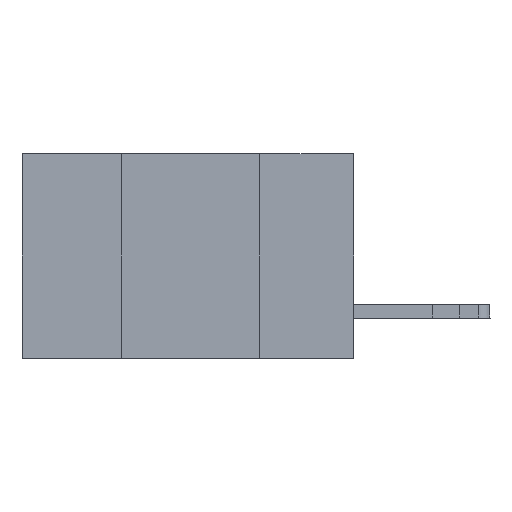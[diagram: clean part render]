
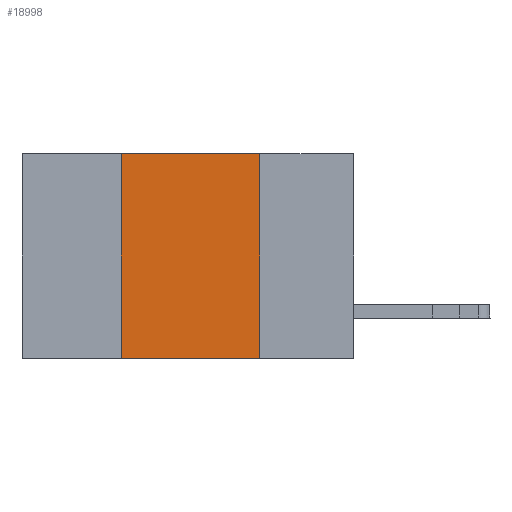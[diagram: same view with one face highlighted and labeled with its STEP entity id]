
A CAD part, left-side view. The second image highlights one B-rep face of the part: STEP entity #18998.
In plain terms, the highlighted planar face has unit normal (-1, 0, 0).
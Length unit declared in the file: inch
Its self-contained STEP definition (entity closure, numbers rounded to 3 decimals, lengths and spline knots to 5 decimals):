
#473 = LINE ( 'NONE', #11415, #4688 ) ;
#1109 = EDGE_CURVE ( 'NONE', #12487, #18572, #7419, .T. ) ;
#1153 = VERTEX_POINT ( 'NONE', #19826 ) ;
#2046 = ORIENTED_EDGE ( 'NONE', *, *, #14550, .T. ) ;
#2418 = CARTESIAN_POINT ( 'NONE',  ( 0., 0.6, -0.37 ) ) ;
#3760 = EDGE_LOOP ( 'NONE', ( #18674, #7766, #18654, #2046 ) ) ;
#4688 = VECTOR ( 'NONE', #9713, 39.37008 ) ;
#5817 = CARTESIAN_POINT ( 'NONE',  ( 0., 0.6, 0. ) ) ;
#6160 = CARTESIAN_POINT ( 'NONE',  ( 0., 0.17, 0. ) ) ;
#6747 = CARTESIAN_POINT ( 'NONE',  ( 0., 0.42, 0. ) ) ;
#7419 = LINE ( 'NONE', #18653, #14099 ) ;
#7720 = FACE_OUTER_BOUND ( 'NONE', #3760, .T. ) ;
#7766 = ORIENTED_EDGE ( 'NONE', *, *, #1109, .F. ) ;
#9285 = DIRECTION ( 'NONE',  ( 0., 0., 1. ) ) ;
#9713 = DIRECTION ( 'NONE',  ( 0., 0., -1. ) ) ;
#10589 = DIRECTION ( 'NONE',  ( 0., -1., 0. ) ) ;
#11415 = CARTESIAN_POINT ( 'NONE',  ( 0., 0.17, 0. ) ) ;
#11754 = DIRECTION ( 'NONE',  ( 0., -1., 0. ) ) ;
#12403 = DIRECTION ( 'NONE',  ( 1., 0., 0. ) ) ;
#12446 = EDGE_CURVE ( 'NONE', #18572, #1153, #473, .T. ) ;
#12487 = VERTEX_POINT ( 'NONE', #6747 ) ;
#13216 = VERTEX_POINT ( 'NONE', #14109 ) ;
#13246 = VECTOR ( 'NONE', #9285, 39.37008 ) ;
#14099 = VECTOR ( 'NONE', #11754, 39.37008 ) ;
#14109 = CARTESIAN_POINT ( 'NONE',  ( 0., 0.42, -0.37 ) ) ;
#14481 = CARTESIAN_POINT ( 'NONE',  ( 0., 0.42, 0. ) ) ;
#14550 = EDGE_CURVE ( 'NONE', #13216, #1153, #16963, .T. ) ;
#15010 = AXIS2_PLACEMENT_3D ( 'NONE', #5817, #12403, #17267 ) ;
#15126 = EDGE_CURVE ( 'NONE', #13216, #12487, #15857, .T. ) ;
#15359 = PLANE ( 'NONE',  #15010 ) ;
#15857 = LINE ( 'NONE', #14481, #13246 ) ;
#16963 = LINE ( 'NONE', #2418, #20357 ) ;
#17267 = DIRECTION ( 'NONE',  ( 0., 0., -1. ) ) ;
#18572 = VERTEX_POINT ( 'NONE', #6160 ) ;
#18653 = CARTESIAN_POINT ( 'NONE',  ( 0., 0.6, 0. ) ) ;
#18654 = ORIENTED_EDGE ( 'NONE', *, *, #15126, .F. ) ;
#18674 = ORIENTED_EDGE ( 'NONE', *, *, #12446, .F. ) ;
#18998 = ADVANCED_FACE ( 'NONE', ( #7720 ), #15359, .F. ) ;
#19826 = CARTESIAN_POINT ( 'NONE',  ( 0., 0.17, -0.37 ) ) ;
#20357 = VECTOR ( 'NONE', #10589, 39.37008 ) ;
